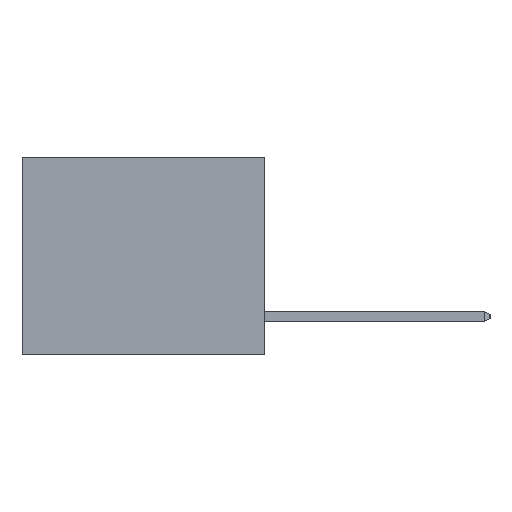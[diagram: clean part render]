
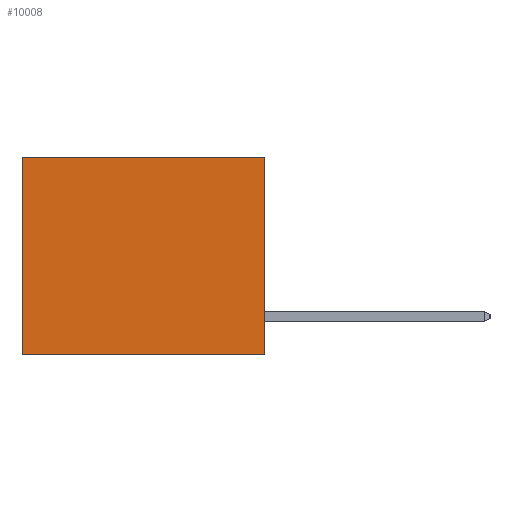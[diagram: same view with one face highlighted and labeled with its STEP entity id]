
A CAD part, left-side view. The second image highlights one B-rep face of the part: STEP entity #10008.
In plain terms, the highlighted planar face has unit normal (-1, 0, 0).
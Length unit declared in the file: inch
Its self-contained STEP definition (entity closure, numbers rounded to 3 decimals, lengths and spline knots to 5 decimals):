
#507 = VERTEX_POINT ( 'NONE', #16612 ) ;
#896 = CARTESIAN_POINT ( 'NONE',  ( 0.3165, 0., -0.49 ) ) ;
#1480 = DIRECTION ( 'NONE',  ( 0., 1., 0. ) ) ;
#1935 = VERTEX_POINT ( 'NONE', #23384 ) ;
#2511 = LINE ( 'NONE', #25638, #7602 ) ;
#2600 = FACE_OUTER_BOUND ( 'NONE', #4219, .T. ) ;
#3225 = DIRECTION ( 'NONE',  ( 0., 0., -1. ) ) ;
#4219 = EDGE_LOOP ( 'NONE', ( #25442, #21250, #25889, #8019 ) ) ;
#5591 = VERTEX_POINT ( 'NONE', #16193 ) ;
#6991 = EDGE_CURVE ( 'NONE', #5591, #1935, #19117, .T. ) ;
#7602 = VECTOR ( 'NONE', #12271, 39.37008 ) ;
#8019 = ORIENTED_EDGE ( 'NONE', *, *, #12263, .T. ) ;
#10008 = ADVANCED_FACE ( 'NONE', ( #2600 ), #24793, .F. ) ;
#10239 = VECTOR ( 'NONE', #20364, 39.37008 ) ;
#10580 = VERTEX_POINT ( 'NONE', #20215 ) ;
#11571 = LINE ( 'NONE', #896, #19411 ) ;
#11895 = DIRECTION ( 'NONE',  ( 0., 0., -1. ) ) ;
#12263 = EDGE_CURVE ( 'NONE', #10580, #5591, #23092, .T. ) ;
#12271 = DIRECTION ( 'NONE',  ( 0., 1., 0. ) ) ;
#13223 = AXIS2_PLACEMENT_3D ( 'NONE', #16230, #16321, #3225 ) ;
#14699 = CARTESIAN_POINT ( 'NONE',  ( 0.3165, 0., 0. ) ) ;
#16193 = CARTESIAN_POINT ( 'NONE',  ( 0.3165, 0.6, 0. ) ) ;
#16230 = CARTESIAN_POINT ( 'NONE',  ( 0.3165, 0., -0.49 ) ) ;
#16321 = DIRECTION ( 'NONE',  ( 1., 0., 0. ) ) ;
#16612 = CARTESIAN_POINT ( 'NONE',  ( 0.3165, 0., -0.49 ) ) ;
#19117 = LINE ( 'NONE', #27261, #10239 ) ;
#19411 = VECTOR ( 'NONE', #11895, 39.37008 ) ;
#20215 = CARTESIAN_POINT ( 'NONE',  ( 0.3165, 0., 0. ) ) ;
#20364 = DIRECTION ( 'NONE',  ( 0., 0., -1. ) ) ;
#21250 = ORIENTED_EDGE ( 'NONE', *, *, #24934, .F. ) ;
#23092 = LINE ( 'NONE', #14699, #24458 ) ;
#23384 = CARTESIAN_POINT ( 'NONE',  ( 0.3165, 0.6, -0.49 ) ) ;
#24458 = VECTOR ( 'NONE', #1480, 39.37008 ) ;
#24793 = PLANE ( 'NONE',  #13223 ) ;
#24934 = EDGE_CURVE ( 'NONE', #507, #1935, #2511, .T. ) ;
#25442 = ORIENTED_EDGE ( 'NONE', *, *, #6991, .T. ) ;
#25638 = CARTESIAN_POINT ( 'NONE',  ( 0.3165, 0., -0.49 ) ) ;
#25889 = ORIENTED_EDGE ( 'NONE', *, *, #27035, .F. ) ;
#27035 = EDGE_CURVE ( 'NONE', #10580, #507, #11571, .T. ) ;
#27261 = CARTESIAN_POINT ( 'NONE',  ( 0.3165, 0.6, -0.49 ) ) ;
